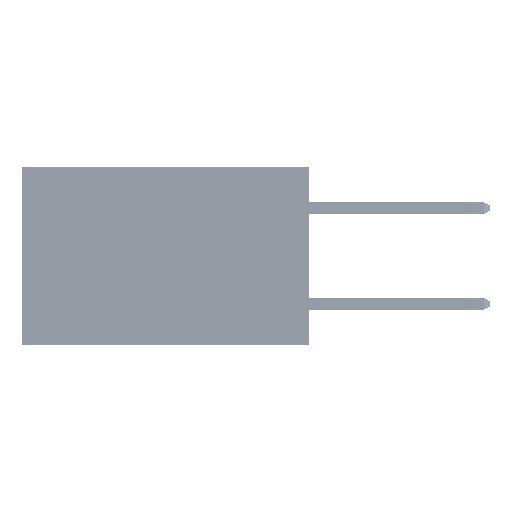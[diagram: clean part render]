
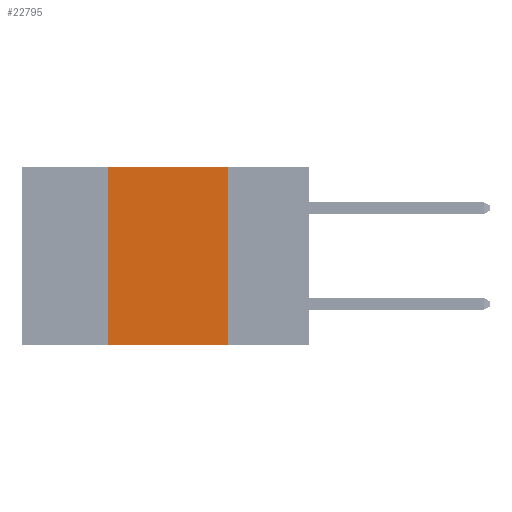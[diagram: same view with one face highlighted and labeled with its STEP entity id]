
A CAD part, left-side view. The second image highlights one B-rep face of the part: STEP entity #22795.
In plain terms, the highlighted planar face has unit normal (-1, 0, 0).
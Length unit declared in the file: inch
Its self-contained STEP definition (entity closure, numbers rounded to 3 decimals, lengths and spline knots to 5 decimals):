
#1475 = LINE ( 'NONE', #24528, #36218 ) ;
#1780 = FACE_OUTER_BOUND ( 'NONE', #11426, .T. ) ;
#2017 = VERTEX_POINT ( 'NONE', #43603 ) ;
#3591 = LINE ( 'NONE', #24265, #45917 ) ;
#4566 = VERTEX_POINT ( 'NONE', #23176 ) ;
#5435 = CARTESIAN_POINT ( 'NONE',  ( 0., 0.6, 0. ) ) ;
#5456 = EDGE_CURVE ( 'NONE', #2017, #42913, #25415, .T. ) ;
#5501 = CARTESIAN_POINT ( 'NONE',  ( 0., 0.6, 0. ) ) ;
#9109 = PLANE ( 'NONE',  #32499 ) ;
#10565 = LINE ( 'NONE', #45956, #29226 ) ;
#11426 = EDGE_LOOP ( 'NONE', ( #39975, #33102, #17902, #13768 ) ) ;
#13768 = ORIENTED_EDGE ( 'NONE', *, *, #29876, .T. ) ;
#17902 = ORIENTED_EDGE ( 'NONE', *, *, #30634, .F. ) ;
#18003 = DIRECTION ( 'NONE',  ( 1., 0., 0. ) ) ;
#22795 = ADVANCED_FACE ( 'NONE', ( #1780 ), #9109, .F. ) ;
#23176 = CARTESIAN_POINT ( 'NONE',  ( 0., 0.17, -0.37 ) ) ;
#23491 = DIRECTION ( 'NONE',  ( 0., -1., 0. ) ) ;
#24265 = CARTESIAN_POINT ( 'NONE',  ( 0., 0.6, -0.37 ) ) ;
#24528 = CARTESIAN_POINT ( 'NONE',  ( 0., 0.17, 0. ) ) ;
#25415 = LINE ( 'NONE', #5501, #49116 ) ;
#29226 = VECTOR ( 'NONE', #46474, 39.37008 ) ;
#29876 = EDGE_CURVE ( 'NONE', #38656, #4566, #3591, .T. ) ;
#30634 = EDGE_CURVE ( 'NONE', #38656, #2017, #10565, .T. ) ;
#32499 = AXIS2_PLACEMENT_3D ( 'NONE', #5435, #18003, #45817 ) ;
#33102 = ORIENTED_EDGE ( 'NONE', *, *, #5456, .F. ) ;
#35375 = DIRECTION ( 'NONE',  ( 0., -1., 0. ) ) ;
#36218 = VECTOR ( 'NONE', #40527, 39.37008 ) ;
#38656 = VERTEX_POINT ( 'NONE', #49387 ) ;
#39975 = ORIENTED_EDGE ( 'NONE', *, *, #48901, .F. ) ;
#40527 = DIRECTION ( 'NONE',  ( 0., 0., -1. ) ) ;
#40635 = CARTESIAN_POINT ( 'NONE',  ( 0., 0.17, 0. ) ) ;
#42913 = VERTEX_POINT ( 'NONE', #40635 ) ;
#43603 = CARTESIAN_POINT ( 'NONE',  ( 0., 0.42, 0. ) ) ;
#45817 = DIRECTION ( 'NONE',  ( 0., 0., -1. ) ) ;
#45917 = VECTOR ( 'NONE', #23491, 39.37008 ) ;
#45956 = CARTESIAN_POINT ( 'NONE',  ( 0., 0.42, 0. ) ) ;
#46474 = DIRECTION ( 'NONE',  ( 0., 0., 1. ) ) ;
#48901 = EDGE_CURVE ( 'NONE', #42913, #4566, #1475, .T. ) ;
#49116 = VECTOR ( 'NONE', #35375, 39.37008 ) ;
#49387 = CARTESIAN_POINT ( 'NONE',  ( 0., 0.42, -0.37 ) ) ;
